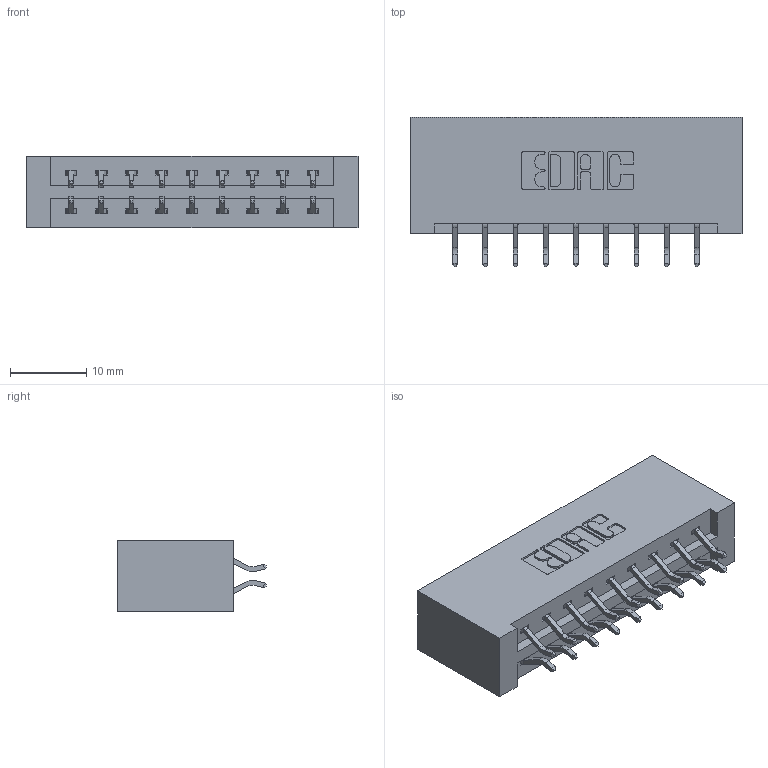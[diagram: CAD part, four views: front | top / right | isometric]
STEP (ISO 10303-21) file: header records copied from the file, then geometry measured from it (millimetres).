
FILE_DESCRIPTION (( 'STEP AP203' ), '1' );
FILE_NAME ('387-018-556-201.STEP', '2019-10-16T01:50:08', ( '' ), ( '' ), 'SwSTEP 2.0', 'SolidWorks 2016', '' );
FILE_SCHEMA (( 'CONFIG_CONTROL_DESIGN' ));
Length unit declared in the file: inch
Products named in the file (3): 345-292-001_556 Tail; 337 Part_No Mounting Lugs; 387-018-556-201
Assembly tree (19 placements, depth 2):
  387-018-556-201
    337 Part_No Mounting Lugs
    345-292-001_556 Tail  x18
Bounding box: 43.54 x 19.57 x 9.4 mm (x, y, z)
Volume: 4908.9 mm3; surface area: 5266.1 mm2
Topology: 19 solids, 19 shells, 1186 faces, 3509 edges, 2314 vertices
Faces by surface type: plane 822, cylinder 364
Entity records: 11189 total; most frequent: CARTESIAN_POINT 1926, ORIENTED_EDGE 1850, DIRECTION 1681, EDGE_CURVE 925, LINE 797, VECTOR 797, VERTEX_POINT 614, AXIS2_PLACEMENT_3D 442
